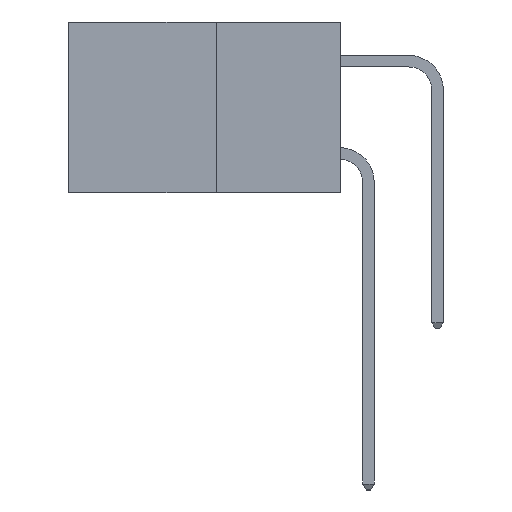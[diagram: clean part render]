
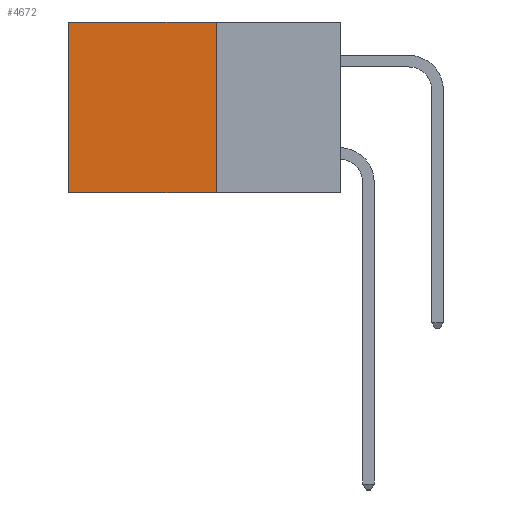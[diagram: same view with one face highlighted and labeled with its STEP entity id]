
A CAD part, left-side view. The second image highlights one B-rep face of the part: STEP entity #4672.
In plain terms, the highlighted planar face has unit normal (-1, 0, 0).
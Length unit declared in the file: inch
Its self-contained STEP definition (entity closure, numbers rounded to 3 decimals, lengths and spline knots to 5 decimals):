
#72 = CARTESIAN_POINT ( 'NONE',  ( 0.277, 0.59, 0. ) ) ;
#509 = CARTESIAN_POINT ( 'NONE',  ( 0.277, 0.27, -0.37 ) ) ;
#595 = VECTOR ( 'NONE', #938, 39.37008 ) ;
#938 = DIRECTION ( 'NONE',  ( 0., 0., -1. ) ) ;
#1005 = EDGE_CURVE ( 'NONE', #1529, #2734, #3284, .T. ) ;
#1168 = DIRECTION ( 'NONE',  ( 0., 1., 0. ) ) ;
#1177 = EDGE_CURVE ( 'NONE', #1529, #8890, #11584, .T. ) ;
#1529 = VERTEX_POINT ( 'NONE', #11655 ) ;
#2734 = VERTEX_POINT ( 'NONE', #10258 ) ;
#3284 = LINE ( 'NONE', #8916, #595 ) ;
#3500 = DIRECTION ( 'NONE',  ( 1., 0., 0. ) ) ;
#3617 = VERTEX_POINT ( 'NONE', #11459 ) ;
#3945 = EDGE_CURVE ( 'NONE', #8890, #3617, #9016, .T. ) ;
#4672 = ADVANCED_FACE ( 'NONE', ( #10779 ), #9707, .F. ) ;
#4879 = AXIS2_PLACEMENT_3D ( 'NONE', #9657, #3500, #9697 ) ;
#4937 = VECTOR ( 'NONE', #12059, 39.37008 ) ;
#5271 = LINE ( 'NONE', #509, #9728 ) ;
#6611 = EDGE_CURVE ( 'NONE', #2734, #3617, #5271, .T. ) ;
#6639 = CARTESIAN_POINT ( 'NONE',  ( 0.277, 0.59, -0.37 ) ) ;
#6828 = DIRECTION ( 'NONE',  ( 0., 0., -1. ) ) ;
#8715 = VECTOR ( 'NONE', #6828, 39.37008 ) ;
#8890 = VERTEX_POINT ( 'NONE', #72 ) ;
#8916 = CARTESIAN_POINT ( 'NONE',  ( 0.277, 0.27, -0.37 ) ) ;
#9016 = LINE ( 'NONE', #6639, #8715 ) ;
#9368 = ORIENTED_EDGE ( 'NONE', *, *, #3945, .T. ) ;
#9391 = ORIENTED_EDGE ( 'NONE', *, *, #6611, .F. ) ;
#9657 = CARTESIAN_POINT ( 'NONE',  ( 0.277, 0.27, -0.37 ) ) ;
#9687 = ORIENTED_EDGE ( 'NONE', *, *, #1005, .F. ) ;
#9697 = DIRECTION ( 'NONE',  ( 0., 0., -1. ) ) ;
#9707 = PLANE ( 'NONE',  #4879 ) ;
#9728 = VECTOR ( 'NONE', #1168, 39.37008 ) ;
#9893 = CARTESIAN_POINT ( 'NONE',  ( 0.277, 0.27, 0. ) ) ;
#10067 = EDGE_LOOP ( 'NONE', ( #9368, #9391, #9687, #10306 ) ) ;
#10258 = CARTESIAN_POINT ( 'NONE',  ( 0.277, 0.27, -0.37 ) ) ;
#10306 = ORIENTED_EDGE ( 'NONE', *, *, #1177, .T. ) ;
#10779 = FACE_OUTER_BOUND ( 'NONE', #10067, .T. ) ;
#11459 = CARTESIAN_POINT ( 'NONE',  ( 0.277, 0.59, -0.37 ) ) ;
#11584 = LINE ( 'NONE', #9893, #4937 ) ;
#11655 = CARTESIAN_POINT ( 'NONE',  ( 0.277, 0.27, 0. ) ) ;
#12059 = DIRECTION ( 'NONE',  ( 0., 1., 0. ) ) ;
